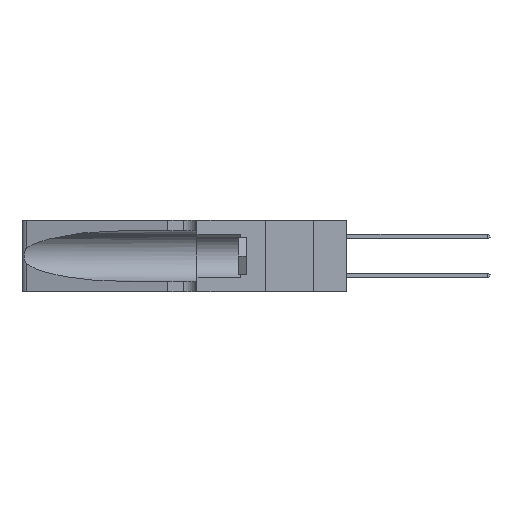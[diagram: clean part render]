
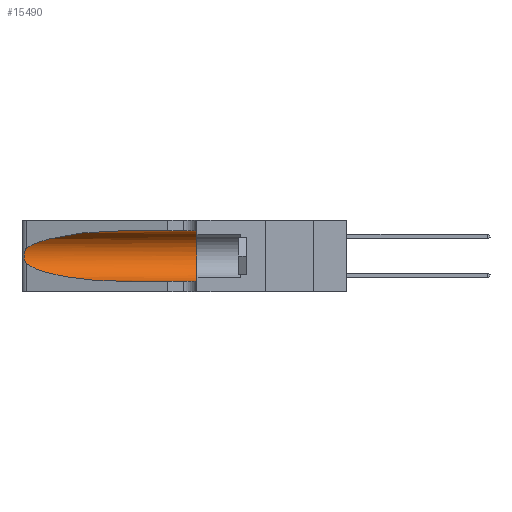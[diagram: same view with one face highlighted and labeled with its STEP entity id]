
A CAD part, left-side view. The second image highlights one B-rep face of the part: STEP entity #15490.
In plain terms, the highlighted cylindrical face has radius 3.308 mm (diameter 6.617 mm), a partial arc.
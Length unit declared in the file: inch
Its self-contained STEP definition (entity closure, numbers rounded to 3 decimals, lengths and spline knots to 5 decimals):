
#394 = CARTESIAN_POINT ( 'NONE',  ( 0.1305, 1.61858, 0.185 ) ) ;
#902 = CARTESIAN_POINT ( 'NONE',  ( 0.25487, 1.22718, 0.14631 ) ) ;
#1706 = CARTESIAN_POINT ( 'NONE',  ( 0.26017, 1.23833, 0.17102 ) ) ;
#2465 = ORIENTED_EDGE ( 'NONE', *, *, #6183, .T. ) ;
#2777 = EDGE_CURVE ( 'NONE', #20046, #19656, #19583, .T. ) ;
#3307 = CARTESIAN_POINT ( 'NONE',  ( 0.18966, 0.96281, 0.05475 ) ) ;
#3513 = DIRECTION ( 'NONE',  ( 0., -1., 0. ) ) ;
#3767 = CARTESIAN_POINT ( 'NONE',  ( 0.25639, 1.23184, 0.21858 ) ) ;
#3859 = CARTESIAN_POINT ( 'NONE',  ( 0.25789, 1.23486, 0.15765 ) ) ;
#3989 = CARTESIAN_POINT ( 'NONE',  ( 0.1305, 0.72297, 0.31525 ) ) ;
#4159 = CARTESIAN_POINT ( 'NONE',  ( 0.1305, 0.35, 0.05475 ) ) ;
#4762 = CYLINDRICAL_SURFACE ( 'NONE', #9018, 0.13025 ) ;
#5168 = DIRECTION ( 'NONE',  ( 0., 1., 0. ) ) ;
#5997 = CARTESIAN_POINT ( 'NONE',  ( 0.25555, 1.22993, 0.14849 ) ) ;
#6183 = EDGE_CURVE ( 'NONE', #11167, #25048, #18632, .T. ) ;
#6599 = LINE ( 'NONE', #7690, #22644 ) ;
#7403 = EDGE_CURVE ( 'NONE', #24469, #20046, #6599, .T. ) ;
#7651 = CARTESIAN_POINT ( 'NONE',  ( 0.1305, 0.72297, 0.31525 ) ) ;
#7690 = CARTESIAN_POINT ( 'NONE',  ( 0.1305, 1.61858, 0.31525 ) ) ;
#8033 = CARTESIAN_POINT ( 'NONE',  ( 0.25487, 1.22718, 0.22369 ) ) ;
#8242 = CARTESIAN_POINT ( 'NONE',  ( 0.25487, 1.22718, 0.22369 ) ) ;
#8911 =( BOUNDED_CURVE ( )  B_SPLINE_CURVE ( 3, ( #22129, #20027, #3307, #17990 ),
 .UNSPECIFIED., .F., .T. ) 
 B_SPLINE_CURVE_WITH_KNOTS ( ( 4, 4 ),
 ( 3.44316, 4.71239 ),
 .UNSPECIFIED. ) 
 CURVE ( )  GEOMETRIC_REPRESENTATION_ITEM ( )  RATIONAL_B_SPLINE_CURVE ( ( 1., 0.87, 0.87, 1. ) ) 
 REPRESENTATION_ITEM ( '' )  );
#9018 = AXIS2_PLACEMENT_3D ( 'NONE', #394, #15163, #13077 ) ;
#10165 = CARTESIAN_POINT ( 'NONE',  ( 0.25787, 1.23484, 0.2124 ) ) ;
#10736 = ORIENTED_EDGE ( 'NONE', *, *, #21073, .T. ) ;
#10892 = EDGE_CURVE ( 'NONE', #25048, #18864, #8911, .T. ) ;
#11167 = VERTEX_POINT ( 'NONE', #23019 ) ;
#11252 = EDGE_CURVE ( 'NONE', #18864, #19656, #11861, .T. ) ;
#11753 =( BOUNDED_CURVE ( )  B_SPLINE_CURVE ( 3, ( #3989, #16543, #20788, #8242 ),
 .UNSPECIFIED., .F., .T. ) 
 B_SPLINE_CURVE_WITH_KNOTS ( ( 4, 4 ),
 ( 1.5708, 2.84003 ),
 .UNSPECIFIED. ) 
 CURVE ( )  GEOMETRIC_REPRESENTATION_ITEM ( )  RATIONAL_B_SPLINE_CURVE ( ( 1., 0.87, 0.87, 1. ) ) 
 REPRESENTATION_ITEM ( '' )  );
#11861 = LINE ( 'NONE', #21567, #22339 ) ;
#12235 = CARTESIAN_POINT ( 'NONE',  ( 0.26018, 1.23835, 0.19895 ) ) ;
#13077 = DIRECTION ( 'NONE',  ( 0., 0., -1. ) ) ;
#13461 = EDGE_LOOP ( 'NONE', ( #10736, #2465, #27220, #13994, #25309, #25408 ) ) ;
#13994 = ORIENTED_EDGE ( 'NONE', *, *, #11252, .T. ) ;
#14332 = CARTESIAN_POINT ( 'NONE',  ( 0.26075, 1.23896, 0.178 ) ) ;
#15163 = DIRECTION ( 'NONE',  ( 0., -1., 0. ) ) ;
#15490 = ADVANCED_FACE ( 'NONE', ( #15904 ), #4762, .F. ) ;
#15904 = FACE_OUTER_BOUND ( 'NONE', #13461, .T. ) ;
#16251 = CARTESIAN_POINT ( 'NONE',  ( 0.25555, 1.22994, 0.2215 ) ) ;
#16421 = CARTESIAN_POINT ( 'NONE',  ( 0.25856, 1.23593, 0.16098 ) ) ;
#16543 = CARTESIAN_POINT ( 'NONE',  ( 0.18966, 0.96281, 0.31525 ) ) ;
#17698 = CARTESIAN_POINT ( 'NONE',  ( 0.1305, 0.35, 0.185 ) ) ;
#17990 = CARTESIAN_POINT ( 'NONE',  ( 0.1305, 0.72297, 0.05475 ) ) ;
#18552 = CARTESIAN_POINT ( 'NONE',  ( 0.25639, 1.23186, 0.15144 ) ) ;
#18632 = B_SPLINE_CURVE_WITH_KNOTS ( 'NONE', 3,
 ( #8033, #16251, #3767, #10165, #24769, #12235, #26864, #14332, #1706, #16421, #3859, #18552, #5997, #20669 ),
 .UNSPECIFIED., .F., .F.,
 ( 4, 2, 2, 2, 2, 2, 4 ),
 ( 0., 0.00027, 0.00053, 0.00107, 0.0016, 0.00187, 0.00214 ),
 .UNSPECIFIED. ) ;
#18864 = VERTEX_POINT ( 'NONE', #26809 ) ;
#19583 = CIRCLE ( 'NONE', #24984, 0.13025 ) ;
#19656 = VERTEX_POINT ( 'NONE', #4159 ) ;
#19832 = DIRECTION ( 'NONE',  ( 0., 0., 1. ) ) ;
#20027 = CARTESIAN_POINT ( 'NONE',  ( 0.2373, 1.15595, 0.08982 ) ) ;
#20046 = VERTEX_POINT ( 'NONE', #20464 ) ;
#20464 = CARTESIAN_POINT ( 'NONE',  ( 0.1305, 0.35, 0.31525 ) ) ;
#20669 = CARTESIAN_POINT ( 'NONE',  ( 0.25487, 1.22718, 0.14631 ) ) ;
#20788 = CARTESIAN_POINT ( 'NONE',  ( 0.2373, 1.15595, 0.28018 ) ) ;
#21073 = EDGE_CURVE ( 'NONE', #24469, #11167, #11753, .T. ) ;
#21567 = CARTESIAN_POINT ( 'NONE',  ( 0.1305, 1.61858, 0.05475 ) ) ;
#22129 = CARTESIAN_POINT ( 'NONE',  ( 0.25487, 1.22718, 0.14631 ) ) ;
#22339 = VECTOR ( 'NONE', #23655, 39.37008 ) ;
#22644 = VECTOR ( 'NONE', #3513, 39.37008 ) ;
#23019 = CARTESIAN_POINT ( 'NONE',  ( 0.25487, 1.22718, 0.22369 ) ) ;
#23655 = DIRECTION ( 'NONE',  ( 0., -1., 0. ) ) ;
#24469 = VERTEX_POINT ( 'NONE', #7651 ) ;
#24769 = CARTESIAN_POINT ( 'NONE',  ( 0.25854, 1.2359, 0.20912 ) ) ;
#24984 = AXIS2_PLACEMENT_3D ( 'NONE', #17698, #5168, #19832 ) ;
#25048 = VERTEX_POINT ( 'NONE', #902 ) ;
#25309 = ORIENTED_EDGE ( 'NONE', *, *, #2777, .F. ) ;
#25408 = ORIENTED_EDGE ( 'NONE', *, *, #7403, .F. ) ;
#26809 = CARTESIAN_POINT ( 'NONE',  ( 0.1305, 0.72297, 0.05475 ) ) ;
#26864 = CARTESIAN_POINT ( 'NONE',  ( 0.26075, 1.23896, 0.19203 ) ) ;
#27220 = ORIENTED_EDGE ( 'NONE', *, *, #10892, .T. ) ;
